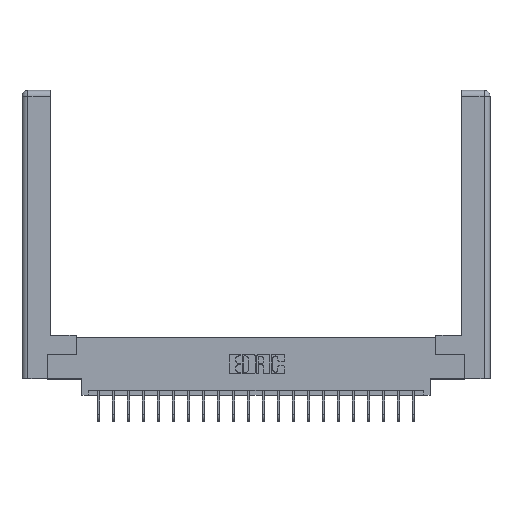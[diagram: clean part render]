
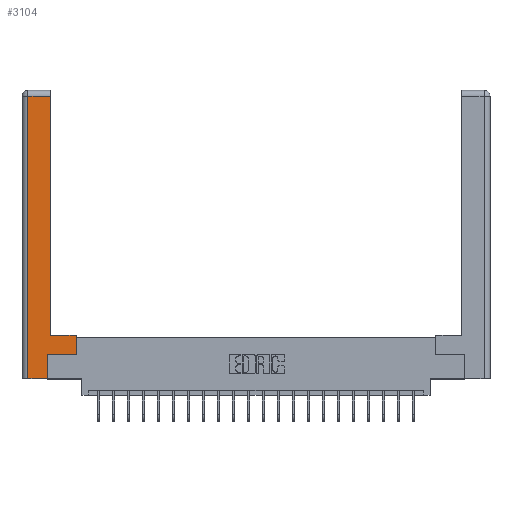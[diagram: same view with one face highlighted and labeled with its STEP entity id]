
A CAD part, top view. The second image highlights one B-rep face of the part: STEP entity #3104.
In plain terms, the highlighted planar face has unit normal (0, 0, 1).
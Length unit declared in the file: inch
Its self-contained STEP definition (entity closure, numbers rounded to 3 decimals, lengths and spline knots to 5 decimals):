
#680 = EDGE_CURVE ( 'NONE', #15403, #9241, #16523, .T. ) ;
#859 = VECTOR ( 'NONE', #21377, 39.37008 ) ;
#999 = VERTEX_POINT ( 'NONE', #3060 ) ;
#1645 = CARTESIAN_POINT ( 'NONE',  ( 0.0615, 0., 0. ) ) ;
#2821 = DIRECTION ( 'NONE',  ( 1., 0., 0. ) ) ;
#3060 = CARTESIAN_POINT ( 'NONE',  ( 0.295, 0.45, 0. ) ) ;
#3077 = EDGE_LOOP ( 'NONE', ( #10015, #7893, #5735, #10739, #20382, #16659, #15559, #5236 ) ) ;
#3104 = ADVANCED_FACE ( 'NONE', ( #3578 ), #8747, .F. ) ;
#3176 = CARTESIAN_POINT ( 'NONE',  ( 0.295, 2.94, 0. ) ) ;
#3578 = FACE_OUTER_BOUND ( 'NONE', #3077, .T. ) ;
#3677 = VECTOR ( 'NONE', #23345, 39.37008 ) ;
#3858 = DIRECTION ( 'NONE',  ( -1., 0., 0. ) ) ;
#4011 = LINE ( 'NONE', #11074, #20964 ) ;
#4487 = DIRECTION ( 'NONE',  ( 0., 1., 0. ) ) ;
#4979 = DIRECTION ( 'NONE',  ( 0., 0., -1. ) ) ;
#4987 = VECTOR ( 'NONE', #2821, 39.37008 ) ;
#5236 = ORIENTED_EDGE ( 'NONE', *, *, #23655, .T. ) ;
#5735 = ORIENTED_EDGE ( 'NONE', *, *, #680, .T. ) ;
#6791 = DIRECTION ( 'NONE',  ( -1., 0., 0. ) ) ;
#7893 = ORIENTED_EDGE ( 'NONE', *, *, #17540, .T. ) ;
#8747 = PLANE ( 'NONE',  #9647 ) ;
#9241 = VERTEX_POINT ( 'NONE', #1645 ) ;
#9476 = CARTESIAN_POINT ( 'NONE',  ( 0.565, 0.245, 0. ) ) ;
#9647 = AXIS2_PLACEMENT_3D ( 'NONE', #20162, #4979, #6791 ) ;
#10015 = ORIENTED_EDGE ( 'NONE', *, *, #21962, .T. ) ;
#10260 = EDGE_CURVE ( 'NONE', #12435, #14735, #12240, .T. ) ;
#10739 = ORIENTED_EDGE ( 'NONE', *, *, #21614, .T. ) ;
#10786 = LINE ( 'NONE', #20306, #18382 ) ;
#11014 = VERTEX_POINT ( 'NONE', #12382 ) ;
#11027 = EDGE_CURVE ( 'NONE', #14735, #16483, #17470, .T. ) ;
#11074 = CARTESIAN_POINT ( 'NONE',  ( 0.295, 0.45, 0. ) ) ;
#12240 = LINE ( 'NONE', #15618, #18397 ) ;
#12382 = CARTESIAN_POINT ( 'NONE',  ( 0.565, 0.45, 0. ) ) ;
#12435 = VERTEX_POINT ( 'NONE', #22735 ) ;
#12504 = VECTOR ( 'NONE', #19695, 39.37008 ) ;
#12516 = LINE ( 'NONE', #17214, #859 ) ;
#12549 = CARTESIAN_POINT ( 'NONE',  ( 0.0615, 2.94, 0. ) ) ;
#12736 = CARTESIAN_POINT ( 'NONE',  ( 0.265, 0.245, 0. ) ) ;
#13127 = LINE ( 'NONE', #21467, #4987 ) ;
#14160 = LINE ( 'NONE', #21552, #3677 ) ;
#14531 = DIRECTION ( 'NONE',  ( 0., 1., 0. ) ) ;
#14735 = VERTEX_POINT ( 'NONE', #12736 ) ;
#15041 = DIRECTION ( 'NONE',  ( 0., -1., 0. ) ) ;
#15403 = VERTEX_POINT ( 'NONE', #12549 ) ;
#15559 = ORIENTED_EDGE ( 'NONE', *, *, #20832, .T. ) ;
#15618 = CARTESIAN_POINT ( 'NONE',  ( 0.265, 0.245, 0. ) ) ;
#16483 = VERTEX_POINT ( 'NONE', #9476 ) ;
#16523 = LINE ( 'NONE', #22575, #18619 ) ;
#16659 = ORIENTED_EDGE ( 'NONE', *, *, #11027, .T. ) ;
#17214 = CARTESIAN_POINT ( 'NONE',  ( 0.565, 0.45, 0. ) ) ;
#17470 = LINE ( 'NONE', #21921, #12504 ) ;
#17540 = EDGE_CURVE ( 'NONE', #18590, #15403, #14160, .T. ) ;
#18382 = VECTOR ( 'NONE', #14531, 39.37008 ) ;
#18397 = VECTOR ( 'NONE', #4487, 39.37008 ) ;
#18590 = VERTEX_POINT ( 'NONE', #3176 ) ;
#18619 = VECTOR ( 'NONE', #15041, 39.37008 ) ;
#19695 = DIRECTION ( 'NONE',  ( 1., 0., 0. ) ) ;
#20162 = CARTESIAN_POINT ( 'NONE',  ( 0., 0., 0. ) ) ;
#20306 = CARTESIAN_POINT ( 'NONE',  ( 0.295, 3., 0. ) ) ;
#20382 = ORIENTED_EDGE ( 'NONE', *, *, #10260, .T. ) ;
#20832 = EDGE_CURVE ( 'NONE', #16483, #11014, #12516, .T. ) ;
#20964 = VECTOR ( 'NONE', #3858, 39.37008 ) ;
#21377 = DIRECTION ( 'NONE',  ( 0., 1., 0. ) ) ;
#21467 = CARTESIAN_POINT ( 'NONE',  ( 0.265, 0., 0. ) ) ;
#21552 = CARTESIAN_POINT ( 'NONE',  ( 0.0615, 2.94, 0. ) ) ;
#21614 = EDGE_CURVE ( 'NONE', #9241, #12435, #13127, .T. ) ;
#21921 = CARTESIAN_POINT ( 'NONE',  ( 0.565, 0.245, 0. ) ) ;
#21962 = EDGE_CURVE ( 'NONE', #999, #18590, #10786, .T. ) ;
#22575 = CARTESIAN_POINT ( 'NONE',  ( 0.0615, 0., 0. ) ) ;
#22735 = CARTESIAN_POINT ( 'NONE',  ( 0.265, 0., 0. ) ) ;
#23345 = DIRECTION ( 'NONE',  ( -1., 0., 0. ) ) ;
#23655 = EDGE_CURVE ( 'NONE', #11014, #999, #4011, .T. ) ;
